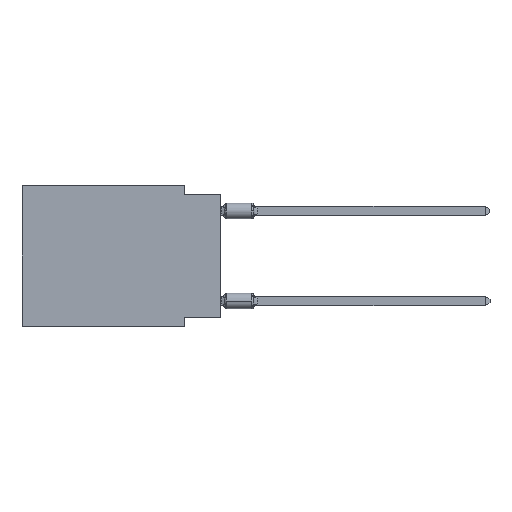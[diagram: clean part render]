
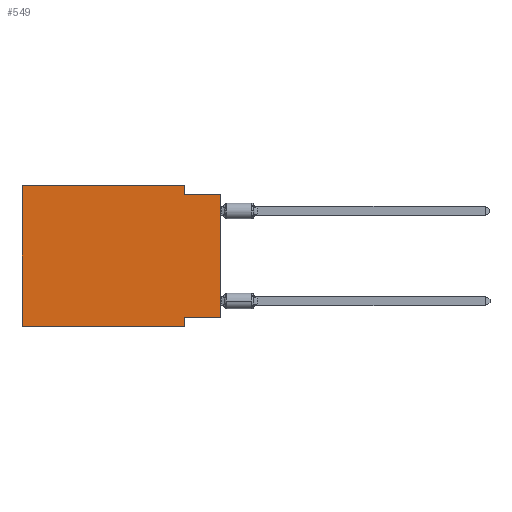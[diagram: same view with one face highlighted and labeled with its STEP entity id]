
A CAD part, left-side view. The second image highlights one B-rep face of the part: STEP entity #549.
In plain terms, the highlighted planar face has unit normal (-1, 0, 0).
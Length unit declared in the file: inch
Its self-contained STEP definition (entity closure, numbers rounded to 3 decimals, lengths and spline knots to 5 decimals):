
#74 = ORIENTED_EDGE ( 'NONE', *, *, #6603, .F. ) ;
#111 = CARTESIAN_POINT ( 'NONE',  ( 0., 0.55, -0.39 ) ) ;
#135 = DIRECTION ( 'NONE',  ( 0., 0., -1. ) ) ;
#164 = VERTEX_POINT ( 'NONE', #9558 ) ;
#400 = ORIENTED_EDGE ( 'NONE', *, *, #3268, .F. ) ;
#441 = DIRECTION ( 'NONE',  ( 0., 0., -1. ) ) ;
#541 = VECTOR ( 'NONE', #12110, 39.37008 ) ;
#549 = ADVANCED_FACE ( 'NONE', ( #5301 ), #4567, .F. ) ;
#1165 = LINE ( 'NONE', #2213, #541 ) ;
#1471 = CARTESIAN_POINT ( 'NONE',  ( 0., 0.1, 0. ) ) ;
#1945 = CARTESIAN_POINT ( 'NONE',  ( 0., 0., 0. ) ) ;
#2213 = CARTESIAN_POINT ( 'NONE',  ( 0., 0.1, -0.39 ) ) ;
#2469 = DIRECTION ( 'NONE',  ( 0., -1., 0. ) ) ;
#2677 = EDGE_CURVE ( 'NONE', #9647, #11996, #6767, .T. ) ;
#2787 = VECTOR ( 'NONE', #10761, 39.37008 ) ;
#3268 = EDGE_CURVE ( 'NONE', #164, #10767, #1165, .T. ) ;
#3328 = CARTESIAN_POINT ( 'NONE',  ( 0., 0.55, 0. ) ) ;
#3520 = DIRECTION ( 'NONE',  ( 0., 1., 0. ) ) ;
#3581 = LINE ( 'NONE', #7652, #5697 ) ;
#3725 = CARTESIAN_POINT ( 'NONE',  ( 0., 0.55, 0. ) ) ;
#3980 = EDGE_CURVE ( 'NONE', #9647, #10767, #9947, .T. ) ;
#4181 = DIRECTION ( 'NONE',  ( 0., -1., 0. ) ) ;
#4498 = EDGE_CURVE ( 'NONE', #11996, #8278, #11239, .T. ) ;
#4567 = PLANE ( 'NONE',  #10648 ) ;
#4737 = CARTESIAN_POINT ( 'NONE',  ( 0., 0.55, 0. ) ) ;
#5301 = FACE_OUTER_BOUND ( 'NONE', #10635, .T. ) ;
#5359 = CARTESIAN_POINT ( 'NONE',  ( 0., 0.55, 0. ) ) ;
#5396 = LINE ( 'NONE', #9325, #11777 ) ;
#5697 = VECTOR ( 'NONE', #3520, 39.37008 ) ;
#5901 = VERTEX_POINT ( 'NONE', #12363 ) ;
#5941 = EDGE_CURVE ( 'NONE', #5901, #164, #3581, .T. ) ;
#5945 = DIRECTION ( 'NONE',  ( 0., 0., 1. ) ) ;
#6603 = EDGE_CURVE ( 'NONE', #8278, #9784, #5396, .T. ) ;
#6767 = LINE ( 'NONE', #4737, #2787 ) ;
#7155 = VECTOR ( 'NONE', #4181, 39.37008 ) ;
#7184 = DIRECTION ( 'NONE',  ( 0., -1., 0. ) ) ;
#7301 = ORIENTED_EDGE ( 'NONE', *, *, #3980, .T. ) ;
#7464 = DIRECTION ( 'NONE',  ( 1., 0., 0. ) ) ;
#7652 = CARTESIAN_POINT ( 'NONE',  ( 0., 0., -0.365 ) ) ;
#8204 = VECTOR ( 'NONE', #7184, 39.37008 ) ;
#8264 = ORIENTED_EDGE ( 'NONE', *, *, #12935, .F. ) ;
#8278 = VERTEX_POINT ( 'NONE', #1471 ) ;
#8415 = VECTOR ( 'NONE', #2469, 39.37008 ) ;
#8749 = CARTESIAN_POINT ( 'NONE',  ( 0., 0.1, -0.025 ) ) ;
#9325 = CARTESIAN_POINT ( 'NONE',  ( 0., 0.1, 0. ) ) ;
#9476 = CARTESIAN_POINT ( 'NONE',  ( 0., 0., -0.025 ) ) ;
#9482 = CARTESIAN_POINT ( 'NONE',  ( 0., 0., -0.025 ) ) ;
#9558 = CARTESIAN_POINT ( 'NONE',  ( 0., 0.1, -0.365 ) ) ;
#9647 = VERTEX_POINT ( 'NONE', #10264 ) ;
#9728 = VERTEX_POINT ( 'NONE', #9482 ) ;
#9784 = VERTEX_POINT ( 'NONE', #8749 ) ;
#9933 = LINE ( 'NONE', #1945, #11762 ) ;
#9946 = ORIENTED_EDGE ( 'NONE', *, *, #2677, .F. ) ;
#9947 = LINE ( 'NONE', #111, #7155 ) ;
#10264 = CARTESIAN_POINT ( 'NONE',  ( 0., 0.55, -0.39 ) ) ;
#10635 = EDGE_LOOP ( 'NONE', ( #11888, #8264, #74, #12640, #9946, #7301, #400, #11832 ) ) ;
#10648 = AXIS2_PLACEMENT_3D ( 'NONE', #3328, #7464, #441 ) ;
#10761 = DIRECTION ( 'NONE',  ( 0., 0., 1. ) ) ;
#10767 = VERTEX_POINT ( 'NONE', #12366 ) ;
#11239 = LINE ( 'NONE', #5359, #8204 ) ;
#11762 = VECTOR ( 'NONE', #5945, 39.37008 ) ;
#11777 = VECTOR ( 'NONE', #135, 39.37008 ) ;
#11832 = ORIENTED_EDGE ( 'NONE', *, *, #5941, .F. ) ;
#11888 = ORIENTED_EDGE ( 'NONE', *, *, #12659, .T. ) ;
#11996 = VERTEX_POINT ( 'NONE', #3725 ) ;
#12110 = DIRECTION ( 'NONE',  ( 0., 0., -1. ) ) ;
#12363 = CARTESIAN_POINT ( 'NONE',  ( 0., 0., -0.365 ) ) ;
#12366 = CARTESIAN_POINT ( 'NONE',  ( 0., 0.1, -0.39 ) ) ;
#12629 = LINE ( 'NONE', #9476, #8415 ) ;
#12640 = ORIENTED_EDGE ( 'NONE', *, *, #4498, .F. ) ;
#12659 = EDGE_CURVE ( 'NONE', #5901, #9728, #9933, .T. ) ;
#12935 = EDGE_CURVE ( 'NONE', #9784, #9728, #12629, .T. ) ;
